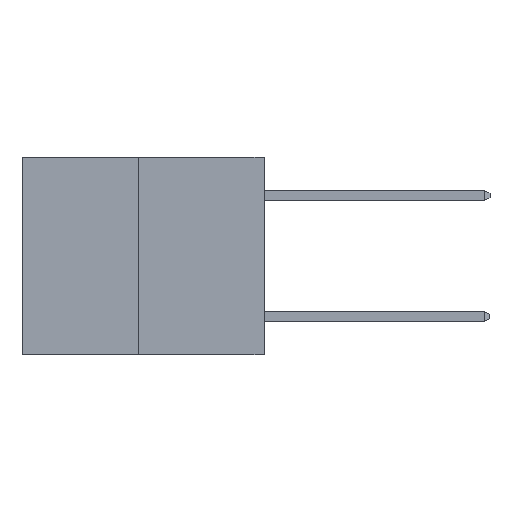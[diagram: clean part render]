
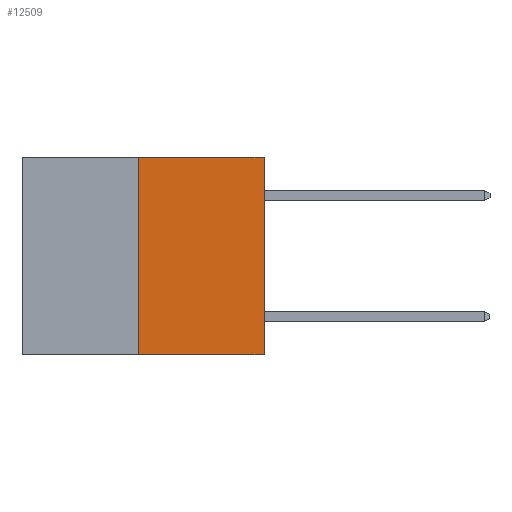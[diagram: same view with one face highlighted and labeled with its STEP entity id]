
A CAD part, left-side view. The second image highlights one B-rep face of the part: STEP entity #12509.
In plain terms, the highlighted planar face has unit normal (-1, 0, 0).
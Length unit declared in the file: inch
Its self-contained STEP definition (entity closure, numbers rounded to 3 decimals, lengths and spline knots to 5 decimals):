
#386 = EDGE_CURVE ( 'NONE', #3182, #3543, #12985, .T. ) ;
#1947 = LINE ( 'NONE', #10308, #14216 ) ;
#2114 = ORIENTED_EDGE ( 'NONE', *, *, #386, .T. ) ;
#2160 = CARTESIAN_POINT ( 'NONE',  ( 0., 0., 0. ) ) ;
#2170 = CARTESIAN_POINT ( 'NONE',  ( 0., 0.312, -0.49 ) ) ;
#2743 = DIRECTION ( 'NONE',  ( 0., 0., 1. ) ) ;
#3182 = VERTEX_POINT ( 'NONE', #5841 ) ;
#3428 = VECTOR ( 'NONE', #6407, 39.37008 ) ;
#3543 = VERTEX_POINT ( 'NONE', #2160 ) ;
#4092 = ORIENTED_EDGE ( 'NONE', *, *, #11903, .F. ) ;
#4268 = CARTESIAN_POINT ( 'NONE',  ( 0., 0.6, -0.49 ) ) ;
#4544 = VERTEX_POINT ( 'NONE', #14501 ) ;
#4613 = DIRECTION ( 'NONE',  ( 0., 0., -1. ) ) ;
#4725 = CARTESIAN_POINT ( 'NONE',  ( 0., 0.6, 0. ) ) ;
#5033 = DIRECTION ( 'NONE',  ( 0., 0., 1. ) ) ;
#5668 = DIRECTION ( 'NONE',  ( 1., 0., 0. ) ) ;
#5841 = CARTESIAN_POINT ( 'NONE',  ( 0., 0., -0.49 ) ) ;
#6091 = CARTESIAN_POINT ( 'NONE',  ( 0., 0.312, -0.49 ) ) ;
#6129 = ORIENTED_EDGE ( 'NONE', *, *, #10124, .F. ) ;
#6323 = CARTESIAN_POINT ( 'NONE',  ( 0., 0., 0. ) ) ;
#6407 = DIRECTION ( 'NONE',  ( 0., -1., 0. ) ) ;
#6599 = EDGE_LOOP ( 'NONE', ( #6129, #8690, #2114, #4092 ) ) ;
#7410 = VECTOR ( 'NONE', #2743, 39.37008 ) ;
#7760 = DIRECTION ( 'NONE',  ( 0., -1., 0. ) ) ;
#8540 = VERTEX_POINT ( 'NONE', #2170 ) ;
#8690 = ORIENTED_EDGE ( 'NONE', *, *, #11660, .T. ) ;
#9051 = AXIS2_PLACEMENT_3D ( 'NONE', #4725, #5668, #4613 ) ;
#9220 = VECTOR ( 'NONE', #5033, 39.37008 ) ;
#10025 = LINE ( 'NONE', #6091, #7410 ) ;
#10124 = EDGE_CURVE ( 'NONE', #8540, #4544, #10025, .T. ) ;
#10308 = CARTESIAN_POINT ( 'NONE',  ( 0., 0.6, 0. ) ) ;
#10429 = FACE_OUTER_BOUND ( 'NONE', #6599, .T. ) ;
#11660 = EDGE_CURVE ( 'NONE', #8540, #3182, #12920, .T. ) ;
#11867 = PLANE ( 'NONE',  #9051 ) ;
#11903 = EDGE_CURVE ( 'NONE', #4544, #3543, #1947, .T. ) ;
#12509 = ADVANCED_FACE ( 'NONE', ( #10429 ), #11867, .F. ) ;
#12920 = LINE ( 'NONE', #4268, #3428 ) ;
#12985 = LINE ( 'NONE', #6323, #9220 ) ;
#14216 = VECTOR ( 'NONE', #7760, 39.37008 ) ;
#14501 = CARTESIAN_POINT ( 'NONE',  ( 0., 0.312, 0. ) ) ;
